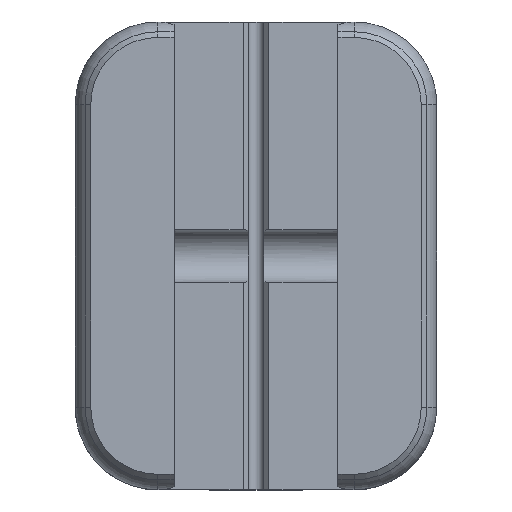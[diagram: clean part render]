
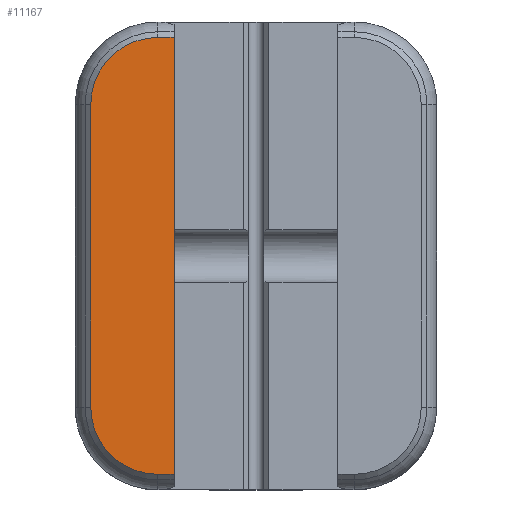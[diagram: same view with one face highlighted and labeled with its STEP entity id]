
A CAD part, top view. The second image highlights one B-rep face of the part: STEP entity #11167.
In plain terms, the highlighted planar face has unit normal (0, 0, 1).
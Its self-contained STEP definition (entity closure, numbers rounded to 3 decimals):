
#199=PLANE('',#12392);
#824=LINE('',#25163,#1371);
#827=LINE('',#25171,#1374);
#838=LINE('',#25198,#1385);
#841=LINE('',#25203,#1388);
#1371=VECTOR('',#15243,10.);
#1374=VECTOR('',#15252,10.);
#1385=VECTOR('',#15281,10.);
#1388=VECTOR('',#15288,10.);
#2348=FACE_OUTER_BOUND('',#3077,.T.);
#3077=EDGE_LOOP('',(#10021,#10022,#10023,#10024,#10025,#10026));
#4190=CIRCLE('',#12376,6.5);
#4191=CIRCLE('',#12379,6.5);
#5128=VERTEX_POINT('',#25155);
#5129=VERTEX_POINT('',#25157);
#5130=VERTEX_POINT('',#25161);
#5131=VERTEX_POINT('',#25165);
#5132=VERTEX_POINT('',#25169);
#5139=VERTEX_POINT('',#25197);
#6768=EDGE_CURVE('',#5128,#5129,#4190,.T.);
#6771=EDGE_CURVE('',#5130,#5128,#824,.T.);
#6773=EDGE_CURVE('',#5131,#5130,#4191,.T.);
#6775=EDGE_CURVE('',#5132,#5131,#827,.T.);
#6789=EDGE_CURVE('',#5129,#5139,#838,.T.);
#6792=EDGE_CURVE('',#5139,#5132,#841,.F.);
#10021=ORIENTED_EDGE('',*,*,#6789,.F.);
#10022=ORIENTED_EDGE('',*,*,#6768,.F.);
#10023=ORIENTED_EDGE('',*,*,#6771,.F.);
#10024=ORIENTED_EDGE('',*,*,#6773,.F.);
#10025=ORIENTED_EDGE('',*,*,#6775,.F.);
#10026=ORIENTED_EDGE('',*,*,#6792,.F.);
#11167=ADVANCED_FACE('',(#2348),#199,.F.);
#12376=AXIS2_PLACEMENT_3D('',#25158,#15237,#15238);
#12379=AXIS2_PLACEMENT_3D('',#25167,#15247,#15248);
#12392=AXIS2_PLACEMENT_3D('',#25205,#15290,#15291);
#15237=DIRECTION('center_axis',(0.,0.,
-1.));
#15238=DIRECTION('ref_axis',(-0.707,0.707,0.));
#15243=DIRECTION('',(0.,1.,0.));
#15247=DIRECTION('center_axis',(0.,0.,
-1.));
#15248=DIRECTION('ref_axis',(-0.707,-0.707,0.));
#15252=DIRECTION('',(-1.,0.,0.));
#15281=DIRECTION('',(1.,0.,0.));
#15288=DIRECTION('',(0.,1.,0.));
#15290=DIRECTION('center_axis',(0.,0.,
-1.));
#15291=DIRECTION('ref_axis',(1.,0.,0.));
#25155=CARTESIAN_POINT('',(-16.,69.653,-24.354));
#25157=CARTESIAN_POINT('',(-9.5,76.153,-24.354));
#25158=CARTESIAN_POINT('Origin',(-9.5,69.653,-24.354));
#25161=CARTESIAN_POINT('',(-16.,40.355,-24.354));
#25163=CARTESIAN_POINT('',(-16.,69.903,-24.354));
#25165=CARTESIAN_POINT('',(-9.5,33.855,-24.354));
#25167=CARTESIAN_POINT('Origin',(-9.5,40.355,-24.354));
#25169=CARTESIAN_POINT('',(-7.936,33.855,-24.354));
#25171=CARTESIAN_POINT('',(-10.135,33.855,-24.354));
#25197=CARTESIAN_POINT('',(-7.936,76.153,-24.354));
#25198=CARTESIAN_POINT('',(-10.135,76.153,-24.354));
#25203=CARTESIAN_POINT('',(-7.936,42.504,-24.354));
#25205=CARTESIAN_POINT('Origin',(-20.269,69.903,-24.354));
